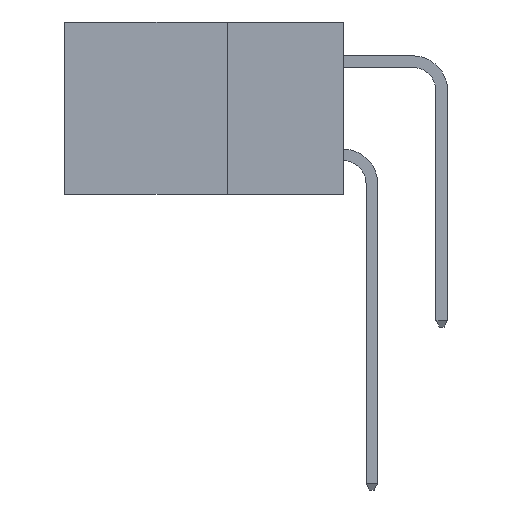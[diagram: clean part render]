
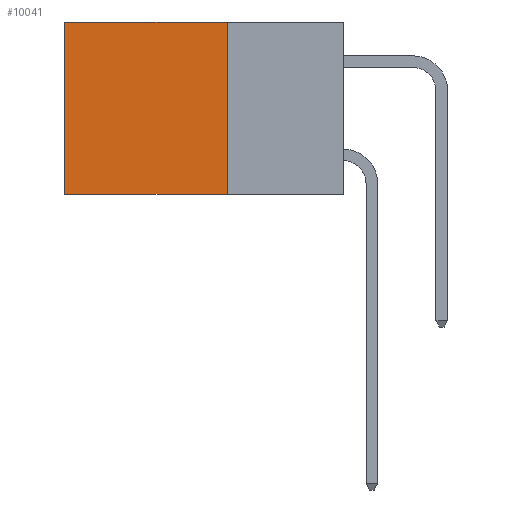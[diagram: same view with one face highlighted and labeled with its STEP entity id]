
A CAD part, left-side view. The second image highlights one B-rep face of the part: STEP entity #10041.
In plain terms, the highlighted planar face has unit normal (-1, 0, 0).
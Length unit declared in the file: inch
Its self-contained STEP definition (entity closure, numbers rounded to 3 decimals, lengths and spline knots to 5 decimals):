
#416 = DIRECTION ( 'NONE',  ( 0., 1., 0. ) ) ;
#514 = CARTESIAN_POINT ( 'NONE',  ( 0.2615, 0.25, 0. ) ) ;
#1050 = VECTOR ( 'NONE', #3526, 39.37008 ) ;
#1286 = EDGE_CURVE ( 'NONE', #1313, #3101, #7614, .T. ) ;
#1313 = VERTEX_POINT ( 'NONE', #15829 ) ;
#1447 = DIRECTION ( 'NONE',  ( 0., 0., -1. ) ) ;
#1448 = DIRECTION ( 'NONE',  ( 1., 0., 0. ) ) ;
#1860 = ORIENTED_EDGE ( 'NONE', *, *, #13398, .F. ) ;
#2201 = CARTESIAN_POINT ( 'NONE',  ( 0.2615, 0.25, -0.37 ) ) ;
#2270 = PLANE ( 'NONE',  #7881 ) ;
#3101 = VERTEX_POINT ( 'NONE', #14058 ) ;
#3397 = VECTOR ( 'NONE', #13860, 39.37008 ) ;
#3526 = DIRECTION ( 'NONE',  ( 0., 1., 0. ) ) ;
#3604 = VERTEX_POINT ( 'NONE', #9396 ) ;
#3684 = EDGE_CURVE ( 'NONE', #3604, #1313, #14514, .T. ) ;
#3785 = CARTESIAN_POINT ( 'NONE',  ( 0.2615, 0.25, -0.37 ) ) ;
#7158 = LINE ( 'NONE', #12517, #3397 ) ;
#7168 = VERTEX_POINT ( 'NONE', #17572 ) ;
#7614 = LINE ( 'NONE', #16117, #10797 ) ;
#7881 = AXIS2_PLACEMENT_3D ( 'NONE', #2201, #1448, #1447 ) ;
#8161 = ORIENTED_EDGE ( 'NONE', *, *, #1286, .T. ) ;
#8922 = FACE_OUTER_BOUND ( 'NONE', #16122, .T. ) ;
#9396 = CARTESIAN_POINT ( 'NONE',  ( 0.2615, 0.25, 0. ) ) ;
#10041 = ADVANCED_FACE ( 'NONE', ( #8922 ), #2270, .F. ) ;
#10797 = VECTOR ( 'NONE', #16059, 39.37008 ) ;
#11816 = VECTOR ( 'NONE', #416, 39.37008 ) ;
#12517 = CARTESIAN_POINT ( 'NONE',  ( 0.2615, 0.25, -0.37 ) ) ;
#13398 = EDGE_CURVE ( 'NONE', #7168, #3101, #15668, .T. ) ;
#13860 = DIRECTION ( 'NONE',  ( 0., 0., -1. ) ) ;
#14024 = ORIENTED_EDGE ( 'NONE', *, *, #3684, .T. ) ;
#14058 = CARTESIAN_POINT ( 'NONE',  ( 0.2615, 0.6, -0.37 ) ) ;
#14514 = LINE ( 'NONE', #514, #11816 ) ;
#15668 = LINE ( 'NONE', #3785, #1050 ) ;
#15829 = CARTESIAN_POINT ( 'NONE',  ( 0.2615, 0.6, 0. ) ) ;
#16059 = DIRECTION ( 'NONE',  ( 0., 0., -1. ) ) ;
#16117 = CARTESIAN_POINT ( 'NONE',  ( 0.2615, 0.6, -0.37 ) ) ;
#16122 = EDGE_LOOP ( 'NONE', ( #8161, #1860, #16930, #14024 ) ) ;
#16930 = ORIENTED_EDGE ( 'NONE', *, *, #17058, .F. ) ;
#17058 = EDGE_CURVE ( 'NONE', #3604, #7168, #7158, .T. ) ;
#17572 = CARTESIAN_POINT ( 'NONE',  ( 0.2615, 0.25, -0.37 ) ) ;
